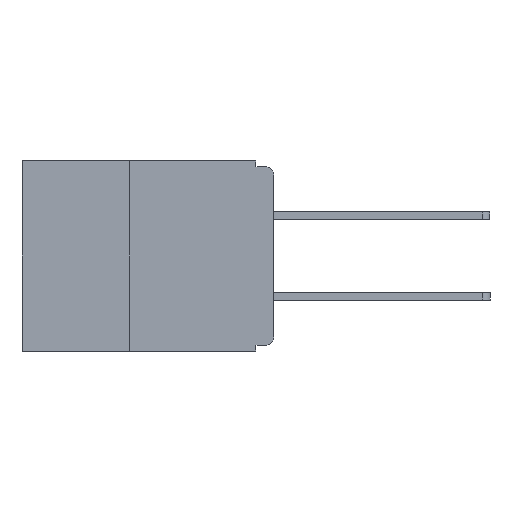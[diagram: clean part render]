
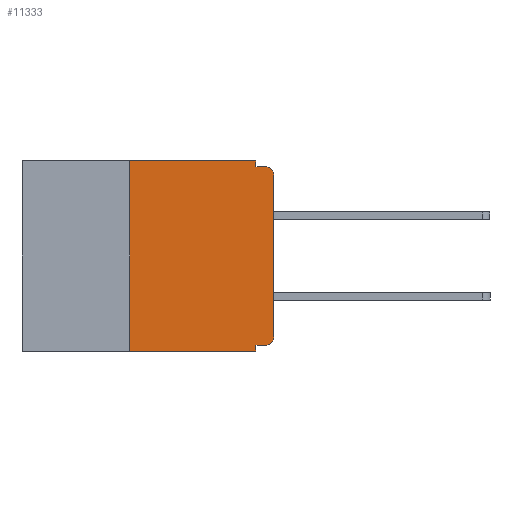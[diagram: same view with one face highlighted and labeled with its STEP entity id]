
A CAD part, left-side view. The second image highlights one B-rep face of the part: STEP entity #11333.
In plain terms, the highlighted planar face has unit normal (-1, 0, 0).
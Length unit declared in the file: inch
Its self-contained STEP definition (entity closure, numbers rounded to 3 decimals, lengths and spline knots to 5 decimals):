
#434 = VERTEX_POINT ( 'NONE', #7120 ) ;
#477 = VERTEX_POINT ( 'NONE', #2674 ) ;
#527 = DIRECTION ( 'NONE',  ( 0., 0., -1. ) ) ;
#548 = EDGE_CURVE ( 'NONE', #4264, #10159, #9547, .T. ) ;
#792 = CARTESIAN_POINT ( 'NONE',  ( 0., 0.015, -0.01 ) ) ;
#804 = EDGE_CURVE ( 'NONE', #477, #4264, #2880, .T. ) ;
#1143 = VERTEX_POINT ( 'NONE', #11665 ) ;
#1334 = ORIENTED_EDGE ( 'NONE', *, *, #15217, .F. ) ;
#1589 = VECTOR ( 'NONE', #4620, 39.37008 ) ;
#1987 = VERTEX_POINT ( 'NONE', #8274 ) ;
#2383 = EDGE_CURVE ( 'NONE', #434, #2590, #12852, .T. ) ;
#2424 = CARTESIAN_POINT ( 'NONE',  ( 0., 0.437, 0. ) ) ;
#2494 = LINE ( 'NONE', #14619, #12331 ) ;
#2565 = ORIENTED_EDGE ( 'NONE', *, *, #15577, .T. ) ;
#2590 = VERTEX_POINT ( 'NONE', #15624 ) ;
#2674 = CARTESIAN_POINT ( 'NONE',  ( 0., 0.25, 0. ) ) ;
#2880 = LINE ( 'NONE', #2424, #16358 ) ;
#3516 = EDGE_CURVE ( 'NONE', #4351, #477, #12448, .T. ) ;
#3740 = CARTESIAN_POINT ( 'NONE',  ( 0., 0.25, -0.33 ) ) ;
#3828 = DIRECTION ( 'NONE',  ( 0., 0., -1. ) ) ;
#3834 = EDGE_CURVE ( 'NONE', #434, #1143, #5073, .T. ) ;
#4033 = DIRECTION ( 'NONE',  ( 0., 0., 1. ) ) ;
#4046 = VECTOR ( 'NONE', #3828, 39.37008 ) ;
#4181 = ORIENTED_EDGE ( 'NONE', *, *, #2383, .F. ) ;
#4264 = VERTEX_POINT ( 'NONE', #5761 ) ;
#4351 = VERTEX_POINT ( 'NONE', #3740 ) ;
#4377 = DIRECTION ( 'NONE',  ( 0., 0., -1. ) ) ;
#4400 = DIRECTION ( 'NONE',  ( -1., 0., 0. ) ) ;
#4429 = VERTEX_POINT ( 'NONE', #792 ) ;
#4432 = CARTESIAN_POINT ( 'NONE',  ( 0., 0.015, -0.305 ) ) ;
#4462 = LINE ( 'NONE', #10222, #4046 ) ;
#4473 = EDGE_CURVE ( 'NONE', #1987, #4429, #12532, .T. ) ;
#4474 = DIRECTION ( 'NONE',  ( 0., -1., 0. ) ) ;
#4620 = DIRECTION ( 'NONE',  ( 0., -1., 0. ) ) ;
#4652 = EDGE_LOOP ( 'NONE', ( #2565, #5112, #6515, #9070, #9495, #11249, #9439, #1334, #4181, #4669 ) ) ;
#4669 = ORIENTED_EDGE ( 'NONE', *, *, #3834, .T. ) ;
#5058 = LINE ( 'NONE', #15913, #1589 ) ;
#5073 = CIRCLE ( 'NONE', #5251, 0.015 ) ;
#5112 = ORIENTED_EDGE ( 'NONE', *, *, #4473, .T. ) ;
#5188 = CARTESIAN_POINT ( 'NONE',  ( 0., 0.25, -0.33 ) ) ;
#5251 = AXIS2_PLACEMENT_3D ( 'NONE', #4432, #4400, #4377 ) ;
#5488 = AXIS2_PLACEMENT_3D ( 'NONE', #16164, #16129, #16077 ) ;
#5704 = DIRECTION ( 'NONE',  ( 0., 1., 0. ) ) ;
#5715 = VECTOR ( 'NONE', #4033, 39.37008 ) ;
#5761 = CARTESIAN_POINT ( 'NONE',  ( 0., 0.031, 0. ) ) ;
#6219 = VECTOR ( 'NONE', #12684, 39.37008 ) ;
#6515 = ORIENTED_EDGE ( 'NONE', *, *, #13164, .F. ) ;
#6860 = DIRECTION ( 'NONE',  ( 0., -1., 0. ) ) ;
#7120 = CARTESIAN_POINT ( 'NONE',  ( 0., 0.015, -0.32 ) ) ;
#7202 = CARTESIAN_POINT ( 'NONE',  ( 0., 0., 0. ) ) ;
#7867 = AXIS2_PLACEMENT_3D ( 'NONE', #13316, #8300, #527 ) ;
#7888 = VECTOR ( 'NONE', #10995, 39.37008 ) ;
#8274 = CARTESIAN_POINT ( 'NONE',  ( 0., 0., -0.025 ) ) ;
#8276 = LINE ( 'NONE', #7202, #7888 ) ;
#8300 = DIRECTION ( 'NONE',  ( 1., 0., 0. ) ) ;
#8337 = CARTESIAN_POINT ( 'NONE',  ( 0., 0.031, -0.01 ) ) ;
#8620 = EDGE_CURVE ( 'NONE', #4351, #10659, #5058, .T. ) ;
#9070 = ORIENTED_EDGE ( 'NONE', *, *, #548, .F. ) ;
#9439 = ORIENTED_EDGE ( 'NONE', *, *, #8620, .T. ) ;
#9495 = ORIENTED_EDGE ( 'NONE', *, *, #804, .F. ) ;
#9547 = LINE ( 'NONE', #11360, #6219 ) ;
#9800 = FACE_OUTER_BOUND ( 'NONE', #4652, .T. ) ;
#9891 = VECTOR ( 'NONE', #5704, 39.37008 ) ;
#10159 = VERTEX_POINT ( 'NONE', #8337 ) ;
#10222 = CARTESIAN_POINT ( 'NONE',  ( 0., 0.031, -0.33 ) ) ;
#10531 = CARTESIAN_POINT ( 'NONE',  ( 0., 0.031, -0.33 ) ) ;
#10659 = VERTEX_POINT ( 'NONE', #10531 ) ;
#10995 = DIRECTION ( 'NONE',  ( 0., 0., 1. ) ) ;
#11249 = ORIENTED_EDGE ( 'NONE', *, *, #3516, .F. ) ;
#11333 = ADVANCED_FACE ( 'NONE', ( #9800 ), #15771, .F. ) ;
#11360 = CARTESIAN_POINT ( 'NONE',  ( 0., 0.031, 0. ) ) ;
#11665 = CARTESIAN_POINT ( 'NONE',  ( 0., 0., -0.305 ) ) ;
#11894 = CARTESIAN_POINT ( 'NONE',  ( 0., 0., -0.32 ) ) ;
#12331 = VECTOR ( 'NONE', #4474, 39.37008 ) ;
#12448 = LINE ( 'NONE', #5188, #5715 ) ;
#12532 = CIRCLE ( 'NONE', #5488, 0.015 ) ;
#12684 = DIRECTION ( 'NONE',  ( 0., 0., -1. ) ) ;
#12852 = LINE ( 'NONE', #11894, #9891 ) ;
#13164 = EDGE_CURVE ( 'NONE', #10159, #4429, #2494, .T. ) ;
#13316 = CARTESIAN_POINT ( 'NONE',  ( 0., 0.437, 0. ) ) ;
#14619 = CARTESIAN_POINT ( 'NONE',  ( 0., 0., -0.01 ) ) ;
#15217 = EDGE_CURVE ( 'NONE', #2590, #10659, #4462, .T. ) ;
#15577 = EDGE_CURVE ( 'NONE', #1143, #1987, #8276, .T. ) ;
#15624 = CARTESIAN_POINT ( 'NONE',  ( 0., 0.031, -0.32 ) ) ;
#15771 = PLANE ( 'NONE',  #7867 ) ;
#15913 = CARTESIAN_POINT ( 'NONE',  ( 0., 0.437, -0.33 ) ) ;
#16077 = DIRECTION ( 'NONE',  ( 0., 0., -1. ) ) ;
#16129 = DIRECTION ( 'NONE',  ( -1., 0., 0. ) ) ;
#16164 = CARTESIAN_POINT ( 'NONE',  ( 0., 0.015, -0.025 ) ) ;
#16358 = VECTOR ( 'NONE', #6860, 39.37008 ) ;
